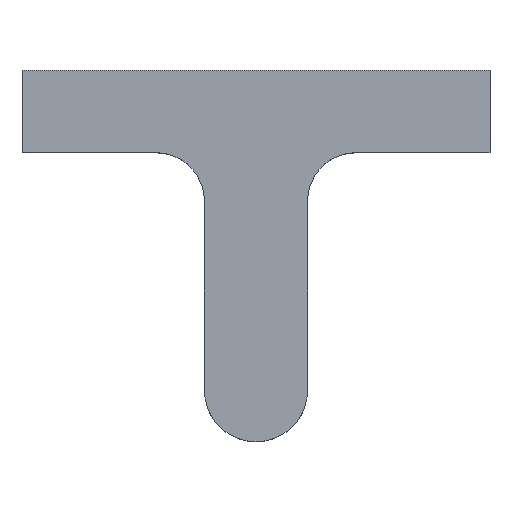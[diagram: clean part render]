
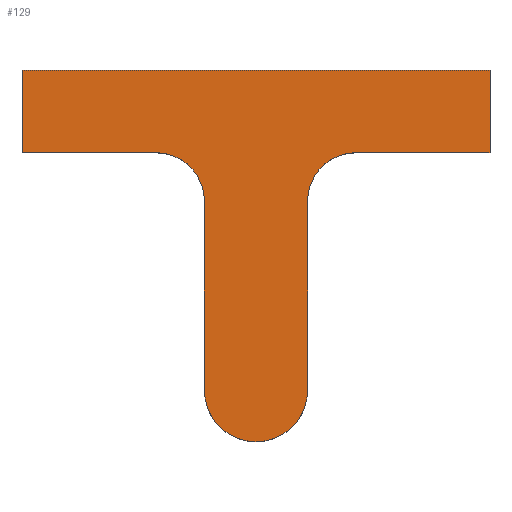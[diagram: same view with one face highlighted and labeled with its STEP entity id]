
A CAD part, top view. The second image highlights one B-rep face of the part: STEP entity #129.
In plain terms, the highlighted planar face has unit normal (0, 0, 1).
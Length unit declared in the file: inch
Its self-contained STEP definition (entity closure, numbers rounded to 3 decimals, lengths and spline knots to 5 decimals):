
#11 = VECTOR ( 'NONE', #284, 39.37008 ) ;
#16 = EDGE_CURVE ( 'NONE', #148, #301, #92, .T. ) ;
#18 = VERTEX_POINT ( 'NONE', #256 ) ;
#19 = VERTEX_POINT ( 'NONE', #33 ) ;
#23 = DIRECTION ( 'NONE',  ( 0., 0., 1. ) ) ;
#28 = CARTESIAN_POINT ( 'NONE',  ( -0.0375, -0.2325, 0.0275 ) ) ;
#33 = CARTESIAN_POINT ( 'NONE',  ( 0.0375, -0.095, 0.0275 ) ) ;
#47 = VECTOR ( 'NONE', #314, 39.37008 ) ;
#49 = ORIENTED_EDGE ( 'NONE', *, *, #398, .T. ) ;
#56 = DIRECTION ( 'NONE',  ( 0., 1., 0. ) ) ;
#60 = EDGE_CURVE ( 'NONE', #169, #238, #258, .T. ) ;
#62 = DIRECTION ( 'NONE',  ( 0., -1., 0. ) ) ;
#63 = LINE ( 'NONE', #85, #47 ) ;
#66 = CARTESIAN_POINT ( 'NONE',  ( 0.0725, -0.06, 0.0275 ) ) ;
#81 = ORIENTED_EDGE ( 'NONE', *, *, #16, .T. ) ;
#82 = ORIENTED_EDGE ( 'NONE', *, *, #91, .T. ) ;
#85 = CARTESIAN_POINT ( 'NONE',  ( 0.17, 0., 0.0275 ) ) ;
#91 = EDGE_CURVE ( 'NONE', #327, #19, #217, .T. ) ;
#92 = LINE ( 'NONE', #127, #219 ) ;
#93 = DIRECTION ( 'NONE',  ( -1., 0., 0. ) ) ;
#97 = CARTESIAN_POINT ( 'NONE',  ( -0.0725, -0.095, 0.0275 ) ) ;
#101 = DIRECTION ( 'NONE',  ( 0., 0., -1. ) ) ;
#104 = VECTOR ( 'NONE', #56, 39.37008 ) ;
#107 = ORIENTED_EDGE ( 'NONE', *, *, #208, .T. ) ;
#113 = VECTOR ( 'NONE', #93, 39.37008 ) ;
#126 = CIRCLE ( 'NONE', #179, 0.035 ) ;
#127 = CARTESIAN_POINT ( 'NONE',  ( -0.17, 0., 0.0275 ) ) ;
#129 = ADVANCED_FACE ( 'NONE', ( #134 ), #318, .F. ) ;
#130 = CARTESIAN_POINT ( 'NONE',  ( 0.0375, -0.2325, 0.0275 ) ) ;
#133 = CARTESIAN_POINT ( 'NONE',  ( -0.17, 0., 0.0275 ) ) ;
#134 = FACE_OUTER_BOUND ( 'NONE', #147, .T. ) ;
#138 = CARTESIAN_POINT ( 'NONE',  ( -0.0725, -0.095, 0.0275 ) ) ;
#139 = EDGE_CURVE ( 'NONE', #303, #169, #126, .T. ) ;
#141 = CIRCLE ( 'NONE', #378, 0.0375 ) ;
#144 = AXIS2_PLACEMENT_3D ( 'NONE', #257, #315, #288 ) ;
#147 = EDGE_LOOP ( 'NONE', ( #81, #107, #331, #276, #202, #82, #49, #358, #401, #149 ) ) ;
#148 = VERTEX_POINT ( 'NONE', #360 ) ;
#149 = ORIENTED_EDGE ( 'NONE', *, *, #414, .T. ) ;
#168 = DIRECTION ( 'NONE',  ( -1., 0., 0. ) ) ;
#169 = VERTEX_POINT ( 'NONE', #226 ) ;
#179 = AXIS2_PLACEMENT_3D ( 'NONE', #97, #101, #168 ) ;
#202 = ORIENTED_EDGE ( 'NONE', *, *, #233, .T. ) ;
#208 = EDGE_CURVE ( 'NONE', #301, #303, #385, .T. ) ;
#210 = VECTOR ( 'NONE', #216, 39.37008 ) ;
#214 = CARTESIAN_POINT ( 'NONE',  ( 0., -0.2325, 0.0275 ) ) ;
#216 = DIRECTION ( 'NONE',  ( 1., 0., 0. ) ) ;
#217 = LINE ( 'NONE', #344, #104 ) ;
#219 = VECTOR ( 'NONE', #62, 39.37008 ) ;
#220 = CARTESIAN_POINT ( 'NONE',  ( -0.17, -0.06, 0.0275 ) ) ;
#221 = CIRCLE ( 'NONE', #144, 0.035 ) ;
#226 = CARTESIAN_POINT ( 'NONE',  ( -0.0375, -0.095, 0.0275 ) ) ;
#231 = AXIS2_PLACEMENT_3D ( 'NONE', #138, #320, #286 ) ;
#233 = EDGE_CURVE ( 'NONE', #238, #327, #141, .T. ) ;
#238 = VERTEX_POINT ( 'NONE', #28 ) ;
#247 = LINE ( 'NONE', #310, #210 ) ;
#249 = CARTESIAN_POINT ( 'NONE',  ( -0.17, -0.06, 0.0275 ) ) ;
#256 = CARTESIAN_POINT ( 'NONE',  ( 0.17, -0.06, 0.0275 ) ) ;
#257 = CARTESIAN_POINT ( 'NONE',  ( 0.0725, -0.095, 0.0275 ) ) ;
#258 = LINE ( 'NONE', #309, #11 ) ;
#264 = EDGE_CURVE ( 'NONE', #371, #18, #247, .T. ) ;
#270 = VERTEX_POINT ( 'NONE', #342 ) ;
#276 = ORIENTED_EDGE ( 'NONE', *, *, #60, .T. ) ;
#284 = DIRECTION ( 'NONE',  ( 0., -1., 0. ) ) ;
#286 = DIRECTION ( 'NONE',  ( -1., 0., 0. ) ) ;
#288 = DIRECTION ( 'NONE',  ( 1., 0., 0. ) ) ;
#301 = VERTEX_POINT ( 'NONE', #249 ) ;
#302 = CARTESIAN_POINT ( 'NONE',  ( -0.0725, -0.06, 0.0275 ) ) ;
#303 = VERTEX_POINT ( 'NONE', #302 ) ;
#309 = CARTESIAN_POINT ( 'NONE',  ( -0.0375, -0.095, 0.0275 ) ) ;
#310 = CARTESIAN_POINT ( 'NONE',  ( 0.17, -0.06, 0.0275 ) ) ;
#314 = DIRECTION ( 'NONE',  ( 0., 1., 0. ) ) ;
#315 = DIRECTION ( 'NONE',  ( 0., 0., -1. ) ) ;
#318 = PLANE ( 'NONE',  #231 ) ;
#320 = DIRECTION ( 'NONE',  ( 0., 0., -1. ) ) ;
#322 = EDGE_CURVE ( 'NONE', #18, #270, #63, .T. ) ;
#327 = VERTEX_POINT ( 'NONE', #130 ) ;
#331 = ORIENTED_EDGE ( 'NONE', *, *, #139, .T. ) ;
#342 = CARTESIAN_POINT ( 'NONE',  ( 0.17, 0., 0.0275 ) ) ;
#344 = CARTESIAN_POINT ( 'NONE',  ( 0.0375, -0.095, 0.0275 ) ) ;
#345 = DIRECTION ( 'NONE',  ( 1., 0., 0. ) ) ;
#358 = ORIENTED_EDGE ( 'NONE', *, *, #264, .T. ) ;
#359 = LINE ( 'NONE', #133, #113 ) ;
#360 = CARTESIAN_POINT ( 'NONE',  ( -0.17, 0., 0.0275 ) ) ;
#371 = VERTEX_POINT ( 'NONE', #66 ) ;
#378 = AXIS2_PLACEMENT_3D ( 'NONE', #214, #23, #409 ) ;
#385 = LINE ( 'NONE', #220, #399 ) ;
#398 = EDGE_CURVE ( 'NONE', #19, #371, #221, .T. ) ;
#399 = VECTOR ( 'NONE', #345, 39.37008 ) ;
#401 = ORIENTED_EDGE ( 'NONE', *, *, #322, .T. ) ;
#409 = DIRECTION ( 'NONE',  ( -1., 0., 0. ) ) ;
#414 = EDGE_CURVE ( 'NONE', #270, #148, #359, .T. ) ;
